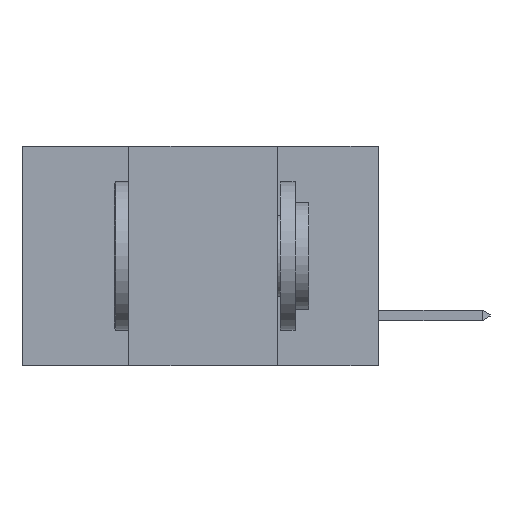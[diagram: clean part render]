
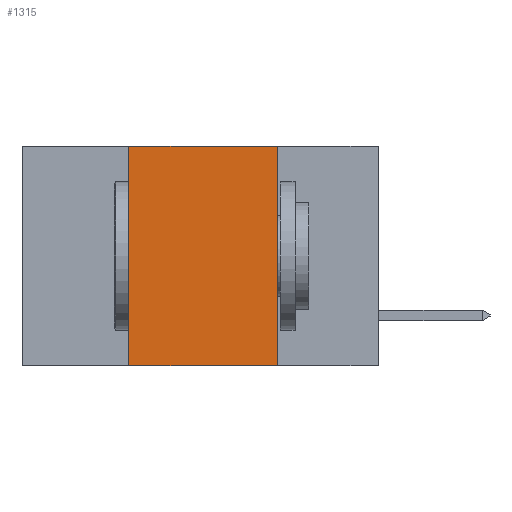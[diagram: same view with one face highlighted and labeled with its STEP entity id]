
A CAD part, left-side view. The second image highlights one B-rep face of the part: STEP entity #1315.
In plain terms, the highlighted planar face has unit normal (-1, 0, 0).
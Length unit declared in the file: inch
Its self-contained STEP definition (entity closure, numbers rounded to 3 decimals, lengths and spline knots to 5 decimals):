
#73 = FACE_OUTER_BOUND ( 'NONE', #584, .T. ) ;
#508 = VECTOR ( 'NONE', #11254, 39.37008 ) ;
#584 = EDGE_LOOP ( 'NONE', ( #11258, #3975, #10987, #2711 ) ) ;
#737 = LINE ( 'NONE', #4472, #2917 ) ;
#1315 = ADVANCED_FACE ( 'NONE', ( #73 ), #7084, .F. ) ;
#1445 = VERTEX_POINT ( 'NONE', #2487 ) ;
#1848 = VERTEX_POINT ( 'NONE', #2687 ) ;
#2487 = CARTESIAN_POINT ( 'NONE',  ( 0., 0.17, -0.37 ) ) ;
#2687 = CARTESIAN_POINT ( 'NONE',  ( 0., 0.42, -0.37 ) ) ;
#2711 = ORIENTED_EDGE ( 'NONE', *, *, #11285, .T. ) ;
#2917 = VECTOR ( 'NONE', #7256, 39.37008 ) ;
#2944 = LINE ( 'NONE', #4922, #7551 ) ;
#3891 = EDGE_CURVE ( 'NONE', #11008, #6665, #7886, .T. ) ;
#3975 = ORIENTED_EDGE ( 'NONE', *, *, #3891, .F. ) ;
#4085 = CARTESIAN_POINT ( 'NONE',  ( 0., 0.17, 0. ) ) ;
#4472 = CARTESIAN_POINT ( 'NONE',  ( 0., 0.6, -0.37 ) ) ;
#4922 = CARTESIAN_POINT ( 'NONE',  ( 0., 0.17, 0. ) ) ;
#4928 = CARTESIAN_POINT ( 'NONE',  ( 0., 0.42, 0. ) ) ;
#5305 = EDGE_CURVE ( 'NONE', #6665, #1445, #2944, .T. ) ;
#5763 = CARTESIAN_POINT ( 'NONE',  ( 0., 0.6, 0. ) ) ;
#6238 = DIRECTION ( 'NONE',  ( 1., 0., 0. ) ) ;
#6357 = DIRECTION ( 'NONE',  ( 0., 0., -1. ) ) ;
#6665 = VERTEX_POINT ( 'NONE', #4085 ) ;
#7084 = PLANE ( 'NONE',  #10933 ) ;
#7256 = DIRECTION ( 'NONE',  ( 0., -1., 0. ) ) ;
#7551 = VECTOR ( 'NONE', #9374, 39.37008 ) ;
#7886 = LINE ( 'NONE', #5763, #508 ) ;
#8018 = EDGE_CURVE ( 'NONE', #1848, #11008, #11287, .T. ) ;
#8335 = CARTESIAN_POINT ( 'NONE',  ( 0., 0.6, 0. ) ) ;
#8919 = VECTOR ( 'NONE', #10618, 39.37008 ) ;
#9374 = DIRECTION ( 'NONE',  ( 0., 0., -1. ) ) ;
#10618 = DIRECTION ( 'NONE',  ( 0., 0., 1. ) ) ;
#10933 = AXIS2_PLACEMENT_3D ( 'NONE', #8335, #6238, #6357 ) ;
#10987 = ORIENTED_EDGE ( 'NONE', *, *, #8018, .F. ) ;
#11008 = VERTEX_POINT ( 'NONE', #4928 ) ;
#11254 = DIRECTION ( 'NONE',  ( 0., -1., 0. ) ) ;
#11258 = ORIENTED_EDGE ( 'NONE', *, *, #5305, .F. ) ;
#11285 = EDGE_CURVE ( 'NONE', #1848, #1445, #737, .T. ) ;
#11287 = LINE ( 'NONE', #11565, #8919 ) ;
#11565 = CARTESIAN_POINT ( 'NONE',  ( 0., 0.42, 0. ) ) ;
